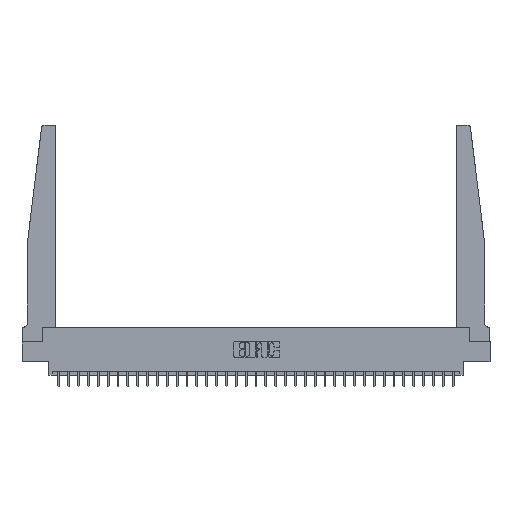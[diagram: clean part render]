
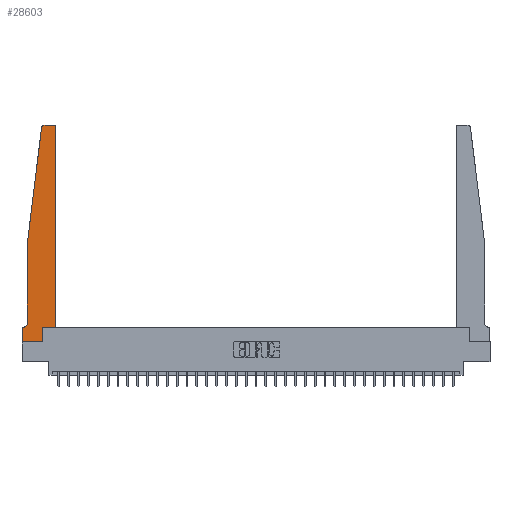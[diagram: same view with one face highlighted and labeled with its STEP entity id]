
A CAD part, top view. The second image highlights one B-rep face of the part: STEP entity #28603.
In plain terms, the highlighted planar face has unit normal (0, 0, 1).
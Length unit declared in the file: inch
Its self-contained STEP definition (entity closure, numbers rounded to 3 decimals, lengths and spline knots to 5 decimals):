
#157 = DIRECTION ( 'NONE',  ( 1., 0., 0. ) ) ;
#160 = DIRECTION ( 'NONE',  ( -1., 0., 0. ) ) ;
#836 = VERTEX_POINT ( 'NONE', #4615 ) ;
#880 = ORIENTED_EDGE ( 'NONE', *, *, #16902, .T. ) ;
#939 = ORIENTED_EDGE ( 'NONE', *, *, #8520, .T. ) ;
#1263 = CARTESIAN_POINT ( 'NONE',  ( 0.395, 2.75, 0.37 ) ) ;
#1337 = CARTESIAN_POINT ( 'NONE',  ( 0.065, 1.25, 0.37 ) ) ;
#1347 = DIRECTION ( 'NONE',  ( 1., 0., 0. ) ) ;
#1683 = VERTEX_POINT ( 'NONE', #6517 ) ;
#2313 = LINE ( 'NONE', #7207, #11003 ) ;
#2517 = EDGE_CURVE ( 'NONE', #17436, #26033, #29609, .T. ) ;
#2545 = CARTESIAN_POINT ( 'NONE',  ( 0.015, 0.1875, 0.37 ) ) ;
#2685 = CIRCLE ( 'NONE', #29794, 0.03 ) ;
#2733 = AXIS2_PLACEMENT_3D ( 'NONE', #28598, #3961, #1347 ) ;
#2906 = CARTESIAN_POINT ( 'NONE',  ( 0.065, 1.25, 0.37 ) ) ;
#3263 = EDGE_CURVE ( 'NONE', #32067, #1683, #24905, .T. ) ;
#3961 = DIRECTION ( 'NONE',  ( 0., 0., 1. ) ) ;
#4033 = CARTESIAN_POINT ( 'NONE',  ( 0.065, 0.2375, 0.37 ) ) ;
#4232 = EDGE_CURVE ( 'NONE', #5139, #20183, #2313, .T. ) ;
#4285 = EDGE_LOOP ( 'NONE', ( #22488, #28662, #5118, #24202, #4471, #27420, #26654, #30232, #29287, #18860, #880, #939 ) ) ;
#4471 = ORIENTED_EDGE ( 'NONE', *, *, #5979, .T. ) ;
#4615 = CARTESIAN_POINT ( 'NONE',  ( 0.2605, 0., 0.37 ) ) ;
#4743 = CARTESIAN_POINT ( 'NONE',  ( 0.25, 2.75, 0.37 ) ) ;
#4854 = CARTESIAN_POINT ( 'NONE',  ( 0.425, 0.18, 0.37 ) ) ;
#4869 = DIRECTION ( 'NONE',  ( 0., 1., 0. ) ) ;
#5026 = LINE ( 'NONE', #10420, #20560 ) ;
#5118 = ORIENTED_EDGE ( 'NONE', *, *, #2517, .T. ) ;
#5139 = VERTEX_POINT ( 'NONE', #24414 ) ;
#5368 = DIRECTION ( 'NONE',  ( 1., 0., 0. ) ) ;
#5979 = EDGE_CURVE ( 'NONE', #19759, #18646, #11716, .T. ) ;
#6018 = EDGE_CURVE ( 'NONE', #18646, #32067, #31678, .T. ) ;
#6517 = CARTESIAN_POINT ( 'NONE',  ( 0., 0., 0.37 ) ) ;
#7207 = CARTESIAN_POINT ( 'NONE',  ( 0.425, 0.18, 0.37 ) ) ;
#7821 = LINE ( 'NONE', #17794, #9987 ) ;
#8520 = EDGE_CURVE ( 'NONE', #10840, #13616, #8794, .T. ) ;
#8794 = CIRCLE ( 'NONE', #14532, 0.03 ) ;
#9987 = VECTOR ( 'NONE', #5368, 39.37008 ) ;
#10420 = CARTESIAN_POINT ( 'NONE',  ( 0.2605, 0.18, 0.37 ) ) ;
#10617 = CARTESIAN_POINT ( 'NONE',  ( 0.395, 2.72, 0.37 ) ) ;
#10840 = VERTEX_POINT ( 'NONE', #30648 ) ;
#11003 = VECTOR ( 'NONE', #27286, 39.37008 ) ;
#11179 = VECTOR ( 'NONE', #14836, 39.37008 ) ;
#11621 = DIRECTION ( 'NONE',  ( -1., 0., 0. ) ) ;
#11716 = CIRCLE ( 'NONE', #24213, 0.05 ) ;
#11884 = EDGE_CURVE ( 'NONE', #26033, #19759, #19091, .T. ) ;
#13363 = DIRECTION ( 'NONE',  ( 0., 0., 1. ) ) ;
#13616 = VERTEX_POINT ( 'NONE', #1263 ) ;
#14018 = VERTEX_POINT ( 'NONE', #24080 ) ;
#14391 = DIRECTION ( 'NONE',  ( 0., 0., -1. ) ) ;
#14532 = AXIS2_PLACEMENT_3D ( 'NONE', #10617, #30518, #157 ) ;
#14836 = DIRECTION ( 'NONE',  ( 0., 1., 0. ) ) ;
#16414 = VECTOR ( 'NONE', #11621, 39.37008 ) ;
#16544 = VECTOR ( 'NONE', #22705, 39.37008 ) ;
#16902 = EDGE_CURVE ( 'NONE', #20183, #10840, #27212, .T. ) ;
#17063 = EDGE_CURVE ( 'NONE', #836, #5139, #5026, .T. ) ;
#17436 = VERTEX_POINT ( 'NONE', #24894 ) ;
#17794 = CARTESIAN_POINT ( 'NONE',  ( 0., 0., 0.37 ) ) ;
#18646 = VERTEX_POINT ( 'NONE', #2545 ) ;
#18735 = DIRECTION ( 'NONE',  ( 1., 0., 0. ) ) ;
#18860 = ORIENTED_EDGE ( 'NONE', *, *, #4232, .T. ) ;
#19091 = LINE ( 'NONE', #2906, #27699 ) ;
#19122 = DIRECTION ( 'NONE',  ( -1., 0., 0. ) ) ;
#19447 = LINE ( 'NONE', #4743, #25475 ) ;
#19759 = VERTEX_POINT ( 'NONE', #4033 ) ;
#20183 = VERTEX_POINT ( 'NONE', #23751 ) ;
#20560 = VECTOR ( 'NONE', #4869, 39.37008 ) ;
#21188 = CARTESIAN_POINT ( 'NONE',  ( 0.27653, 2.72, 0.37 ) ) ;
#21274 = FACE_OUTER_BOUND ( 'NONE', #4285, .T. ) ;
#21441 = VECTOR ( 'NONE', #27518, 39.37008 ) ;
#22488 = ORIENTED_EDGE ( 'NONE', *, *, #22516, .T. ) ;
#22516 = EDGE_CURVE ( 'NONE', #13616, #14018, #19447, .T. ) ;
#22705 = DIRECTION ( 'NONE',  ( -0.122, -0.992, 0. ) ) ;
#23751 = CARTESIAN_POINT ( 'NONE',  ( 0.425, 0.18, 0.37 ) ) ;
#24015 = CARTESIAN_POINT ( 'NONE',  ( 0.065, 0.1875, 0.37 ) ) ;
#24080 = CARTESIAN_POINT ( 'NONE',  ( 0.27653, 2.75, 0.37 ) ) ;
#24202 = ORIENTED_EDGE ( 'NONE', *, *, #11884, .T. ) ;
#24213 = AXIS2_PLACEMENT_3D ( 'NONE', #29244, #14391, #19122 ) ;
#24414 = CARTESIAN_POINT ( 'NONE',  ( 0.2605, 0.18, 0.37 ) ) ;
#24894 = CARTESIAN_POINT ( 'NONE',  ( 0.24675, 2.72367, 0.37 ) ) ;
#24905 = LINE ( 'NONE', #32109, #21441 ) ;
#25475 = VECTOR ( 'NONE', #160, 39.37008 ) ;
#25595 = CARTESIAN_POINT ( 'NONE',  ( 0., 0.1875, 0.37 ) ) ;
#26033 = VERTEX_POINT ( 'NONE', #1337 ) ;
#26654 = ORIENTED_EDGE ( 'NONE', *, *, #3263, .T. ) ;
#27212 = LINE ( 'NONE', #4854, #11179 ) ;
#27286 = DIRECTION ( 'NONE',  ( 1., 0., 0. ) ) ;
#27420 = ORIENTED_EDGE ( 'NONE', *, *, #6018, .T. ) ;
#27518 = DIRECTION ( 'NONE',  ( 0., -1., 0. ) ) ;
#27593 = CARTESIAN_POINT ( 'NONE',  ( 0.065, 1.25, 0.37 ) ) ;
#27699 = VECTOR ( 'NONE', #30010, 39.37008 ) ;
#28598 = CARTESIAN_POINT ( 'NONE',  ( 0., 0.1875, 0.37 ) ) ;
#28603 = ADVANCED_FACE ( 'NONE', ( #21274 ), #31071, .T. ) ;
#28662 = ORIENTED_EDGE ( 'NONE', *, *, #32012, .T. ) ;
#29244 = CARTESIAN_POINT ( 'NONE',  ( 0.015, 0.2375, 0.37 ) ) ;
#29287 = ORIENTED_EDGE ( 'NONE', *, *, #17063, .T. ) ;
#29609 = LINE ( 'NONE', #27593, #16544 ) ;
#29794 = AXIS2_PLACEMENT_3D ( 'NONE', #21188, #13363, #18735 ) ;
#30010 = DIRECTION ( 'NONE',  ( 0., -1., 0. ) ) ;
#30232 = ORIENTED_EDGE ( 'NONE', *, *, #31994, .T. ) ;
#30518 = DIRECTION ( 'NONE',  ( 0., 0., 1. ) ) ;
#30648 = CARTESIAN_POINT ( 'NONE',  ( 0.425, 2.72, 0.37 ) ) ;
#31071 = PLANE ( 'NONE',  #2733 ) ;
#31678 = LINE ( 'NONE', #24015, #16414 ) ;
#31994 = EDGE_CURVE ( 'NONE', #1683, #836, #7821, .T. ) ;
#32012 = EDGE_CURVE ( 'NONE', #14018, #17436, #2685, .T. ) ;
#32067 = VERTEX_POINT ( 'NONE', #25595 ) ;
#32109 = CARTESIAN_POINT ( 'NONE',  ( 0., 0., 0.37 ) ) ;
